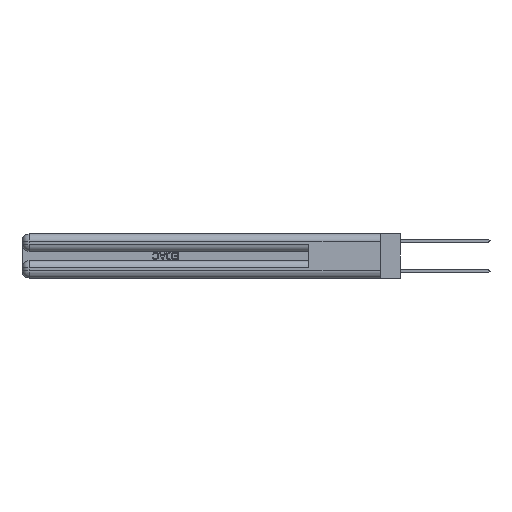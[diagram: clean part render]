
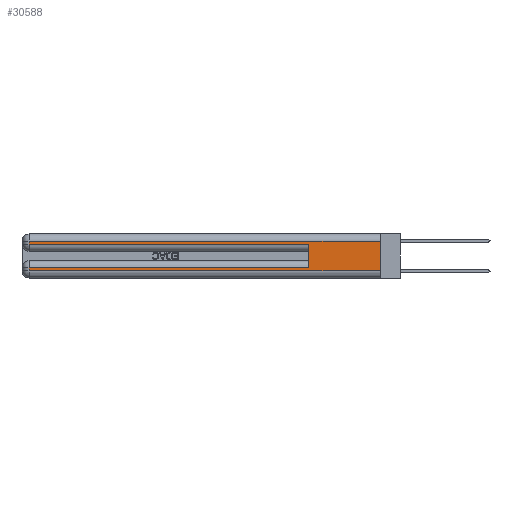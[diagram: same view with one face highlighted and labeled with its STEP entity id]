
A CAD part, left-side view. The second image highlights one B-rep face of the part: STEP entity #30588.
In plain terms, the highlighted planar face has unit normal (-1, 0, 0).
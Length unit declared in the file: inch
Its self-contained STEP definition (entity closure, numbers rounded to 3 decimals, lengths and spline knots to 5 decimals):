
#163 = VERTEX_POINT ( 'NONE', #29567 ) ;
#657 = VECTOR ( 'NONE', #1664, 39.37008 ) ;
#892 = VECTOR ( 'NONE', #26112, 39.37008 ) ;
#1101 = CARTESIAN_POINT ( 'NONE',  ( 0., 0., 0.085 ) ) ;
#1664 = DIRECTION ( 'NONE',  ( 0., 1., 0. ) ) ;
#2015 = DIRECTION ( 'NONE',  ( 0., 0., -1. ) ) ;
#2771 = LINE ( 'NONE', #9038, #3601 ) ;
#3601 = VECTOR ( 'NONE', #27603, 39.37008 ) ;
#4085 = LINE ( 'NONE', #1101, #8670 ) ;
#4440 = ORIENTED_EDGE ( 'NONE', *, *, #17752, .T. ) ;
#5211 = ORIENTED_EDGE ( 'NONE', *, *, #24653, .T. ) ;
#5289 = DIRECTION ( 'NONE',  ( 0., -1., 0. ) ) ;
#5721 = VERTEX_POINT ( 'NONE', #16885 ) ;
#7566 = LINE ( 'NONE', #27299, #20889 ) ;
#7663 = LINE ( 'NONE', #18548, #13891 ) ;
#7864 = VERTEX_POINT ( 'NONE', #26026 ) ;
#7906 = CARTESIAN_POINT ( 'NONE',  ( 0., 2.94, 0.06 ) ) ;
#8670 = VECTOR ( 'NONE', #24992, 39.37008 ) ;
#8737 = DIRECTION ( 'NONE',  ( 0., 0., -1. ) ) ;
#9038 = CARTESIAN_POINT ( 'NONE',  ( 0., 0., 0.37 ) ) ;
#9495 = DIRECTION ( 'NONE',  ( 0., 0., -1. ) ) ;
#9832 = VECTOR ( 'NONE', #9495, 39.37008 ) ;
#9879 = FACE_OUTER_BOUND ( 'NONE', #16583, .T. ) ;
#10272 = EDGE_CURVE ( 'NONE', #7864, #32675, #2771, .T. ) ;
#10704 = AXIS2_PLACEMENT_3D ( 'NONE', #23132, #17902, #2015 ) ;
#12547 = PLANE ( 'NONE',  #10704 ) ;
#12863 = CARTESIAN_POINT ( 'NONE',  ( 0., 0.6, 0.145 ) ) ;
#13024 = VERTEX_POINT ( 'NONE', #20341 ) ;
#13268 = ORIENTED_EDGE ( 'NONE', *, *, #21466, .T. ) ;
#13891 = VECTOR ( 'NONE', #5289, 39.37008 ) ;
#14049 = CARTESIAN_POINT ( 'NONE',  ( 0., 0., 0.06 ) ) ;
#14547 = EDGE_CURVE ( 'NONE', #7864, #13024, #15565, .T. ) ;
#15076 = VERTEX_POINT ( 'NONE', #30829 ) ;
#15565 = LINE ( 'NONE', #17536, #657 ) ;
#16583 = EDGE_LOOP ( 'NONE', ( #19295, #26862, #29283, #4440, #32271, #13268, #33718, #5211 ) ) ;
#16885 = CARTESIAN_POINT ( 'NONE',  ( 0., 0.6, 0.285 ) ) ;
#17150 = EDGE_CURVE ( 'NONE', #163, #5721, #30744, .T. ) ;
#17536 = CARTESIAN_POINT ( 'NONE',  ( 0., 0., 0.31 ) ) ;
#17752 = EDGE_CURVE ( 'NONE', #15076, #5721, #33231, .T. ) ;
#17828 = DIRECTION ( 'NONE',  ( 0., -1., 0. ) ) ;
#17902 = DIRECTION ( 'NONE',  ( 1., 0., 0. ) ) ;
#18548 = CARTESIAN_POINT ( 'NONE',  ( 0., 0., 0.06 ) ) ;
#18850 = EDGE_CURVE ( 'NONE', #13024, #15076, #7566, .T. ) ;
#19295 = ORIENTED_EDGE ( 'NONE', *, *, #10272, .F. ) ;
#20341 = CARTESIAN_POINT ( 'NONE',  ( 0., 2.94, 0.31 ) ) ;
#20889 = VECTOR ( 'NONE', #8737, 39.37008 ) ;
#21466 = EDGE_CURVE ( 'NONE', #163, #31240, #4085, .T. ) ;
#22161 = EDGE_CURVE ( 'NONE', #31240, #28930, #24011, .T. ) ;
#22729 = CARTESIAN_POINT ( 'NONE',  ( 0., 2.94, 0.37 ) ) ;
#23132 = CARTESIAN_POINT ( 'NONE',  ( 0., 0., 0.37 ) ) ;
#24011 = LINE ( 'NONE', #22729, #9832 ) ;
#24653 = EDGE_CURVE ( 'NONE', #28930, #32675, #7663, .T. ) ;
#24992 = DIRECTION ( 'NONE',  ( 0., 1., 0. ) ) ;
#26026 = CARTESIAN_POINT ( 'NONE',  ( 0., 0., 0.31 ) ) ;
#26112 = DIRECTION ( 'NONE',  ( 0., 0., 1. ) ) ;
#26862 = ORIENTED_EDGE ( 'NONE', *, *, #14547, .T. ) ;
#27299 = CARTESIAN_POINT ( 'NONE',  ( 0., 2.94, 0.37 ) ) ;
#27603 = DIRECTION ( 'NONE',  ( 0., 0., -1. ) ) ;
#28075 = CARTESIAN_POINT ( 'NONE',  ( 0., 2.94, 0.085 ) ) ;
#28930 = VERTEX_POINT ( 'NONE', #7906 ) ;
#29283 = ORIENTED_EDGE ( 'NONE', *, *, #18850, .T. ) ;
#29567 = CARTESIAN_POINT ( 'NONE',  ( 0., 0.6, 0.085 ) ) ;
#30588 = ADVANCED_FACE ( 'NONE', ( #9879 ), #12547, .F. ) ;
#30744 = LINE ( 'NONE', #12863, #892 ) ;
#30829 = CARTESIAN_POINT ( 'NONE',  ( 0., 2.94, 0.285 ) ) ;
#31029 = CARTESIAN_POINT ( 'NONE',  ( 0., 0., 0.285 ) ) ;
#31240 = VERTEX_POINT ( 'NONE', #28075 ) ;
#32271 = ORIENTED_EDGE ( 'NONE', *, *, #17150, .F. ) ;
#32422 = VECTOR ( 'NONE', #17828, 39.37008 ) ;
#32675 = VERTEX_POINT ( 'NONE', #14049 ) ;
#33231 = LINE ( 'NONE', #31029, #32422 ) ;
#33718 = ORIENTED_EDGE ( 'NONE', *, *, #22161, .T. ) ;
